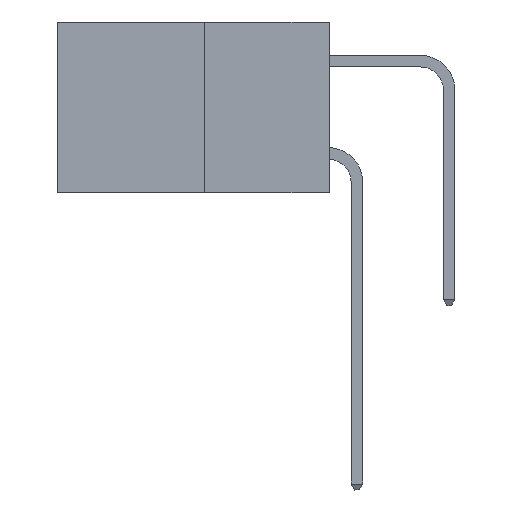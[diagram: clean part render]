
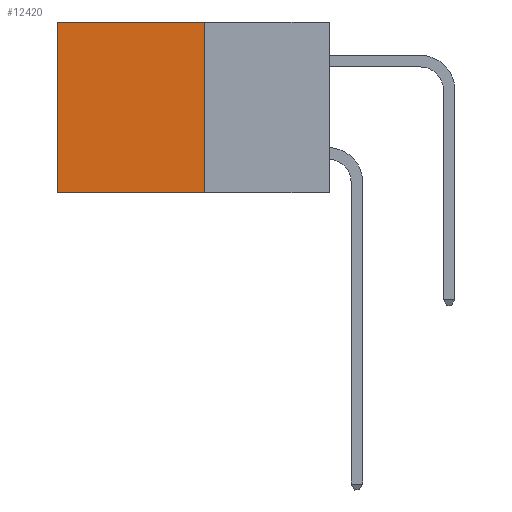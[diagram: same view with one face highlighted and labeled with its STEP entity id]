
A CAD part, left-side view. The second image highlights one B-rep face of the part: STEP entity #12420.
In plain terms, the highlighted planar face has unit normal (-1, 0, 0).
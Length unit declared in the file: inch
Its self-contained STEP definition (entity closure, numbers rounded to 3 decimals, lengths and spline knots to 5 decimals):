
#161 = VERTEX_POINT ( 'NONE', #15718 ) ;
#2904 = EDGE_CURVE ( 'NONE', #13266, #161, #15291, .T. ) ;
#6116 = ORIENTED_EDGE ( 'NONE', *, *, #7638, .T. ) ;
#7638 = EDGE_CURVE ( 'NONE', #13266, #19535, #13626, .T. ) ;
#7824 = VECTOR ( 'NONE', #19278, 39.37008 ) ;
#8074 = CARTESIAN_POINT ( 'NONE',  ( 0.277, 0.27, -0.37 ) ) ;
#10346 = DIRECTION ( 'NONE',  ( 0., 1., 0. ) ) ;
#10406 = CARTESIAN_POINT ( 'NONE',  ( 0.277, 0.27, 0. ) ) ;
#10908 = VECTOR ( 'NONE', #14680, 39.37008 ) ;
#11626 = ORIENTED_EDGE ( 'NONE', *, *, #20215, .F. ) ;
#11875 = AXIS2_PLACEMENT_3D ( 'NONE', #8074, #12660, #28512 ) ;
#12049 = CARTESIAN_POINT ( 'NONE',  ( 0.277, 0.59, 0. ) ) ;
#12406 = CARTESIAN_POINT ( 'NONE',  ( 0.277, 0.59, -0.37 ) ) ;
#12420 = ADVANCED_FACE ( 'NONE', ( #15363 ), #21736, .F. ) ;
#12660 = DIRECTION ( 'NONE',  ( 1., 0., 0. ) ) ;
#13266 = VERTEX_POINT ( 'NONE', #15771 ) ;
#13384 = EDGE_LOOP ( 'NONE', ( #27612, #11626, #27270, #6116 ) ) ;
#13626 = LINE ( 'NONE', #10406, #24297 ) ;
#13880 = LINE ( 'NONE', #14691, #7824 ) ;
#14602 = VECTOR ( 'NONE', #20039, 39.37008 ) ;
#14680 = DIRECTION ( 'NONE',  ( 0., 0., -1. ) ) ;
#14691 = CARTESIAN_POINT ( 'NONE',  ( 0.277, 0.27, -0.37 ) ) ;
#15291 = LINE ( 'NONE', #20071, #14602 ) ;
#15363 = FACE_OUTER_BOUND ( 'NONE', #13384, .T. ) ;
#15718 = CARTESIAN_POINT ( 'NONE',  ( 0.277, 0.27, -0.37 ) ) ;
#15771 = CARTESIAN_POINT ( 'NONE',  ( 0.277, 0.27, 0. ) ) ;
#19278 = DIRECTION ( 'NONE',  ( 0., 1., 0. ) ) ;
#19535 = VERTEX_POINT ( 'NONE', #12049 ) ;
#20039 = DIRECTION ( 'NONE',  ( 0., 0., -1. ) ) ;
#20071 = CARTESIAN_POINT ( 'NONE',  ( 0.277, 0.27, -0.37 ) ) ;
#20215 = EDGE_CURVE ( 'NONE', #161, #26097, #13880, .T. ) ;
#21028 = CARTESIAN_POINT ( 'NONE',  ( 0.277, 0.59, -0.37 ) ) ;
#21436 = EDGE_CURVE ( 'NONE', #19535, #26097, #29015, .T. ) ;
#21736 = PLANE ( 'NONE',  #11875 ) ;
#24297 = VECTOR ( 'NONE', #10346, 39.37008 ) ;
#26097 = VERTEX_POINT ( 'NONE', #21028 ) ;
#27270 = ORIENTED_EDGE ( 'NONE', *, *, #2904, .F. ) ;
#27612 = ORIENTED_EDGE ( 'NONE', *, *, #21436, .T. ) ;
#28512 = DIRECTION ( 'NONE',  ( 0., 0., -1. ) ) ;
#29015 = LINE ( 'NONE', #12406, #10908 ) ;
